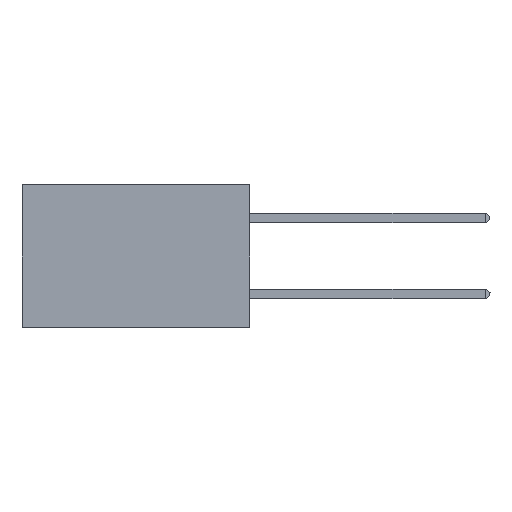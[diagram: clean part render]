
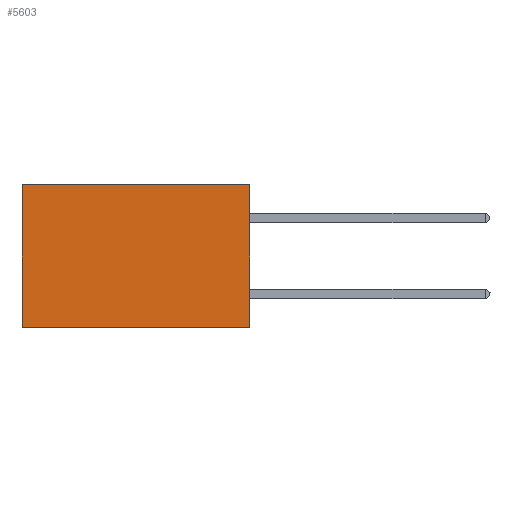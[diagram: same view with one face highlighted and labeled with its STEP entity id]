
A CAD part, left-side view. The second image highlights one B-rep face of the part: STEP entity #5603.
In plain terms, the highlighted planar face has unit normal (-1, 0, 0).
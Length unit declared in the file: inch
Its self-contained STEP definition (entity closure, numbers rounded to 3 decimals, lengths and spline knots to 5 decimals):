
#204 = CARTESIAN_POINT ( 'NONE',  ( 0.2875, 0.6, -0.375 ) ) ;
#297 = EDGE_CURVE ( 'NONE', #16732, #6341, #14304, .T. ) ;
#500 = EDGE_CURVE ( 'NONE', #16732, #7861, #2188, .T. ) ;
#1204 = DIRECTION ( 'NONE',  ( 1., 0., 0. ) ) ;
#1225 = ORIENTED_EDGE ( 'NONE', *, *, #500, .F. ) ;
#1568 = DIRECTION ( 'NONE',  ( 0., 1., 0. ) ) ;
#1838 = CARTESIAN_POINT ( 'NONE',  ( 0.2875, 0., 0. ) ) ;
#2188 = LINE ( 'NONE', #18312, #17680 ) ;
#2787 = CARTESIAN_POINT ( 'NONE',  ( 0.2875, 0., -0.375 ) ) ;
#3223 = DIRECTION ( 'NONE',  ( 0., 0., -1. ) ) ;
#4017 = PLANE ( 'NONE',  #16586 ) ;
#4055 = VECTOR ( 'NONE', #3223, 39.37008 ) ;
#5125 = VECTOR ( 'NONE', #7920, 39.37008 ) ;
#5545 = ORIENTED_EDGE ( 'NONE', *, *, #297, .T. ) ;
#5603 = ADVANCED_FACE ( 'NONE', ( #8582 ), #4017, .F. ) ;
#6341 = VERTEX_POINT ( 'NONE', #13147 ) ;
#7861 = VERTEX_POINT ( 'NONE', #9802 ) ;
#7920 = DIRECTION ( 'NONE',  ( 0., 1., 0. ) ) ;
#8582 = FACE_OUTER_BOUND ( 'NONE', #17611, .T. ) ;
#8802 = CARTESIAN_POINT ( 'NONE',  ( 0.2875, 0.6, -0.375 ) ) ;
#9399 = VECTOR ( 'NONE', #1568, 39.37008 ) ;
#9454 = ORIENTED_EDGE ( 'NONE', *, *, #12351, .F. ) ;
#9802 = CARTESIAN_POINT ( 'NONE',  ( 0.2875, 0., -0.375 ) ) ;
#10799 = CARTESIAN_POINT ( 'NONE',  ( 0.2875, 0., 0. ) ) ;
#11279 = CARTESIAN_POINT ( 'NONE',  ( 0.2875, 0., -0.375 ) ) ;
#12351 = EDGE_CURVE ( 'NONE', #7861, #15310, #16366, .T. ) ;
#13147 = CARTESIAN_POINT ( 'NONE',  ( 0.2875, 0.6, 0. ) ) ;
#13931 = LINE ( 'NONE', #8802, #4055 ) ;
#13932 = DIRECTION ( 'NONE',  ( 0., 0., -1. ) ) ;
#14304 = LINE ( 'NONE', #10799, #5125 ) ;
#15030 = ORIENTED_EDGE ( 'NONE', *, *, #17307, .T. ) ;
#15310 = VERTEX_POINT ( 'NONE', #204 ) ;
#16366 = LINE ( 'NONE', #2787, #9399 ) ;
#16586 = AXIS2_PLACEMENT_3D ( 'NONE', #11279, #1204, #17062 ) ;
#16732 = VERTEX_POINT ( 'NONE', #1838 ) ;
#17062 = DIRECTION ( 'NONE',  ( 0., 0., -1. ) ) ;
#17307 = EDGE_CURVE ( 'NONE', #6341, #15310, #13931, .T. ) ;
#17611 = EDGE_LOOP ( 'NONE', ( #15030, #9454, #1225, #5545 ) ) ;
#17680 = VECTOR ( 'NONE', #13932, 39.37008 ) ;
#18312 = CARTESIAN_POINT ( 'NONE',  ( 0.2875, 0., -0.375 ) ) ;
